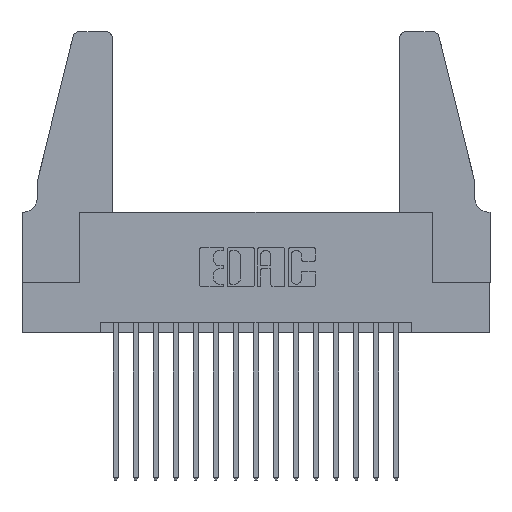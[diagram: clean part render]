
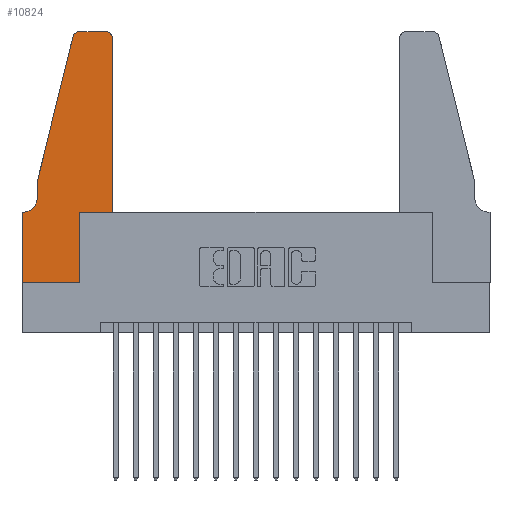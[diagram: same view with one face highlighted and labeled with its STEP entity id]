
A CAD part, top view. The second image highlights one B-rep face of the part: STEP entity #10824.
In plain terms, the highlighted planar face has unit normal (0, 0, 1).
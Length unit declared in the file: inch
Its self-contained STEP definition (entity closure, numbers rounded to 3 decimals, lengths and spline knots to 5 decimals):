
#245 = CARTESIAN_POINT ( 'NONE',  ( 0.2865, 0.35, 0.37 ) ) ;
#349 = CIRCLE ( 'NONE', #2256, 0.07 ) ;
#567 = EDGE_CURVE ( 'NONE', #9430, #3143, #13361, .T. ) ;
#577 = DIRECTION ( 'NONE',  ( -0.239, -0.971, 0. ) ) ;
#865 = CARTESIAN_POINT ( 'NONE',  ( 0.4505, 1.22, 0.37 ) ) ;
#1101 = LINE ( 'NONE', #7027, #15162 ) ;
#1323 = VECTOR ( 'NONE', #5566, 39.37008 ) ;
#1423 = CARTESIAN_POINT ( 'NONE',  ( 0.4505, 0.35, 0.37 ) ) ;
#1562 = LINE ( 'NONE', #1423, #4980 ) ;
#1709 = DIRECTION ( 'NONE',  ( 0., -1., 0. ) ) ;
#1812 = DIRECTION ( 'NONE',  ( 1., 0., 0. ) ) ;
#1903 = CARTESIAN_POINT ( 'NONE',  ( 0.0055, 0.42, 0.37 ) ) ;
#2155 = LINE ( 'NONE', #245, #1323 ) ;
#2256 = AXIS2_PLACEMENT_3D ( 'NONE', #1903, #14012, #3344 ) ;
#2320 = VECTOR ( 'NONE', #13462, 39.37008 ) ;
#2351 = CARTESIAN_POINT ( 'NONE',  ( 0.4505, 0.35, 0.37 ) ) ;
#2666 = VERTEX_POINT ( 'NONE', #17239 ) ;
#2684 = DIRECTION ( 'NONE',  ( 1., 0., 0. ) ) ;
#3087 = CARTESIAN_POINT ( 'NONE',  ( 0.0755, 0.5, 0.37 ) ) ;
#3116 = DIRECTION ( 'NONE',  ( 0., 0., 1. ) ) ;
#3143 = VERTEX_POINT ( 'NONE', #14697 ) ;
#3158 = LINE ( 'NONE', #4868, #10464 ) ;
#3205 = EDGE_CURVE ( 'NONE', #12569, #17473, #2155, .T. ) ;
#3237 = CARTESIAN_POINT ( 'NONE',  ( 0.284, 1.22, 0.37 ) ) ;
#3243 = CARTESIAN_POINT ( 'NONE',  ( 0., 0.35, 0.37 ) ) ;
#3268 = VECTOR ( 'NONE', #6497, 39.37008 ) ;
#3344 = DIRECTION ( 'NONE',  ( -1., 0., 0. ) ) ;
#3527 = CARTESIAN_POINT ( 'NONE',  ( 0.0055, 0.35, 0.37 ) ) ;
#4224 = AXIS2_PLACEMENT_3D ( 'NONE', #16356, #10988, #16299 ) ;
#4272 = ORIENTED_EDGE ( 'NONE', *, *, #4960, .T. ) ;
#4366 = CARTESIAN_POINT ( 'NONE',  ( 0., 0.35, 0.37 ) ) ;
#4451 = ORIENTED_EDGE ( 'NONE', *, *, #6872, .T. ) ;
#4868 = CARTESIAN_POINT ( 'NONE',  ( 0.0755, 0.5, 0.37 ) ) ;
#4960 = EDGE_CURVE ( 'NONE', #17598, #8232, #11876, .T. ) ;
#4980 = VECTOR ( 'NONE', #2684, 39.37008 ) ;
#5509 = EDGE_CURVE ( 'NONE', #8232, #5679, #349, .T. ) ;
#5566 = DIRECTION ( 'NONE',  ( 0., 1., 0. ) ) ;
#5605 = ORIENTED_EDGE ( 'NONE', *, *, #6867, .T. ) ;
#5679 = VERTEX_POINT ( 'NONE', #3527 ) ;
#5781 = LINE ( 'NONE', #6518, #2320 ) ;
#5920 = VECTOR ( 'NONE', #1709, 39.37008 ) ;
#5962 = VERTEX_POINT ( 'NONE', #865 ) ;
#6497 = DIRECTION ( 'NONE',  ( 0., 1., 0. ) ) ;
#6518 = CARTESIAN_POINT ( 'NONE',  ( 0., 0., 0.37 ) ) ;
#6867 = EDGE_CURVE ( 'NONE', #5962, #9430, #7139, .T. ) ;
#6872 = EDGE_CURVE ( 'NONE', #17473, #8707, #1562, .T. ) ;
#7027 = CARTESIAN_POINT ( 'NONE',  ( 0., 0., 0.37 ) ) ;
#7139 = CIRCLE ( 'NONE', #4224, 0.03 ) ;
#7175 = EDGE_LOOP ( 'NONE', ( #14966, #15069, #9998, #4272, #9171, #11277, #13277, #14402, #8032, #4451, #14866, #5605 ) ) ;
#7211 = DIRECTION ( 'NONE',  ( 0., 0., 1. ) ) ;
#7271 = PLANE ( 'NONE',  #11143 ) ;
#8032 = ORIENTED_EDGE ( 'NONE', *, *, #3205, .T. ) ;
#8155 = CARTESIAN_POINT ( 'NONE',  ( 0.0755, 0.5, 0.37 ) ) ;
#8232 = VERTEX_POINT ( 'NONE', #12649 ) ;
#8707 = VERTEX_POINT ( 'NONE', #11219 ) ;
#9171 = ORIENTED_EDGE ( 'NONE', *, *, #5509, .T. ) ;
#9339 = VERTEX_POINT ( 'NONE', #13597 ) ;
#9430 = VERTEX_POINT ( 'NONE', #10170 ) ;
#9451 = CARTESIAN_POINT ( 'NONE',  ( 0.2605, 1.25, 0.37 ) ) ;
#9708 = EDGE_CURVE ( 'NONE', #15314, #9339, #5781, .T. ) ;
#9724 = AXIS2_PLACEMENT_3D ( 'NONE', #3237, #3116, #14133 ) ;
#9998 = ORIENTED_EDGE ( 'NONE', *, *, #10050, .T. ) ;
#10050 = EDGE_CURVE ( 'NONE', #2666, #17598, #3158, .T. ) ;
#10066 = CARTESIAN_POINT ( 'NONE',  ( 0.2865, 0., 0.37 ) ) ;
#10170 = CARTESIAN_POINT ( 'NONE',  ( 0.4205, 1.25, 0.37 ) ) ;
#10464 = VECTOR ( 'NONE', #577, 39.37008 ) ;
#10824 = ADVANCED_FACE ( 'NONE', ( #16497 ), #7271, .T. ) ;
#10988 = DIRECTION ( 'NONE',  ( 0., 0., 1. ) ) ;
#11143 = AXIS2_PLACEMENT_3D ( 'NONE', #3243, #7211, #1812 ) ;
#11219 = CARTESIAN_POINT ( 'NONE',  ( 0.4505, 0.35, 0.37 ) ) ;
#11231 = LINE ( 'NONE', #15136, #11863 ) ;
#11277 = ORIENTED_EDGE ( 'NONE', *, *, #16995, .T. ) ;
#11809 = LINE ( 'NONE', #2351, #3268 ) ;
#11863 = VECTOR ( 'NONE', #12704, 39.37008 ) ;
#11869 = EDGE_CURVE ( 'NONE', #8707, #5962, #11809, .T. ) ;
#11876 = LINE ( 'NONE', #3087, #5920 ) ;
#12569 = VERTEX_POINT ( 'NONE', #10066 ) ;
#12649 = CARTESIAN_POINT ( 'NONE',  ( 0.0755, 0.42, 0.37 ) ) ;
#12704 = DIRECTION ( 'NONE',  ( -1., 0., 0. ) ) ;
#13144 = EDGE_CURVE ( 'NONE', #9339, #12569, #1101, .T. ) ;
#13244 = CIRCLE ( 'NONE', #9724, 0.03 ) ;
#13277 = ORIENTED_EDGE ( 'NONE', *, *, #9708, .T. ) ;
#13291 = EDGE_CURVE ( 'NONE', #3143, #2666, #13244, .T. ) ;
#13361 = LINE ( 'NONE', #9451, #16098 ) ;
#13462 = DIRECTION ( 'NONE',  ( 0., -1., 0. ) ) ;
#13597 = CARTESIAN_POINT ( 'NONE',  ( 0., 0., 0.37 ) ) ;
#14012 = DIRECTION ( 'NONE',  ( 0., 0., -1. ) ) ;
#14133 = DIRECTION ( 'NONE',  ( 1., 0., 0. ) ) ;
#14402 = ORIENTED_EDGE ( 'NONE', *, *, #13144, .T. ) ;
#14697 = CARTESIAN_POINT ( 'NONE',  ( 0.284, 1.25, 0.37 ) ) ;
#14866 = ORIENTED_EDGE ( 'NONE', *, *, #11869, .T. ) ;
#14966 = ORIENTED_EDGE ( 'NONE', *, *, #567, .T. ) ;
#15069 = ORIENTED_EDGE ( 'NONE', *, *, #13291, .T. ) ;
#15136 = CARTESIAN_POINT ( 'NONE',  ( 0.0755, 0.35, 0.37 ) ) ;
#15162 = VECTOR ( 'NONE', #16564, 39.37008 ) ;
#15314 = VERTEX_POINT ( 'NONE', #4366 ) ;
#16098 = VECTOR ( 'NONE', #16101, 39.37008 ) ;
#16101 = DIRECTION ( 'NONE',  ( -1., 0., 0. ) ) ;
#16299 = DIRECTION ( 'NONE',  ( 1., 0., 0. ) ) ;
#16356 = CARTESIAN_POINT ( 'NONE',  ( 0.4205, 1.22, 0.37 ) ) ;
#16497 = FACE_OUTER_BOUND ( 'NONE', #7175, .T. ) ;
#16564 = DIRECTION ( 'NONE',  ( 1., 0., 0. ) ) ;
#16995 = EDGE_CURVE ( 'NONE', #5679, #15314, #11231, .T. ) ;
#17239 = CARTESIAN_POINT ( 'NONE',  ( 0.25487, 1.22718, 0.37 ) ) ;
#17473 = VERTEX_POINT ( 'NONE', #17601 ) ;
#17598 = VERTEX_POINT ( 'NONE', #8155 ) ;
#17601 = CARTESIAN_POINT ( 'NONE',  ( 0.2865, 0.35, 0.37 ) ) ;
